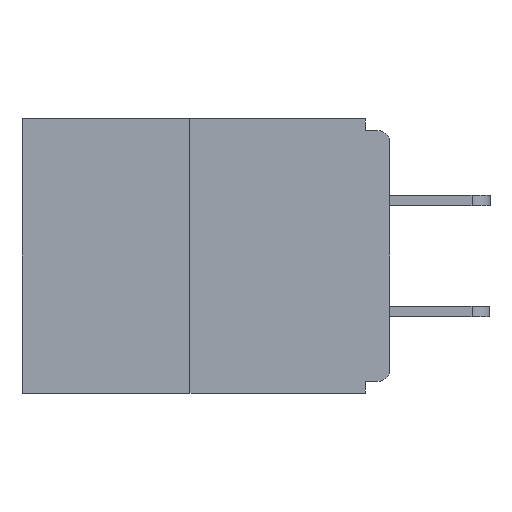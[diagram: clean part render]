
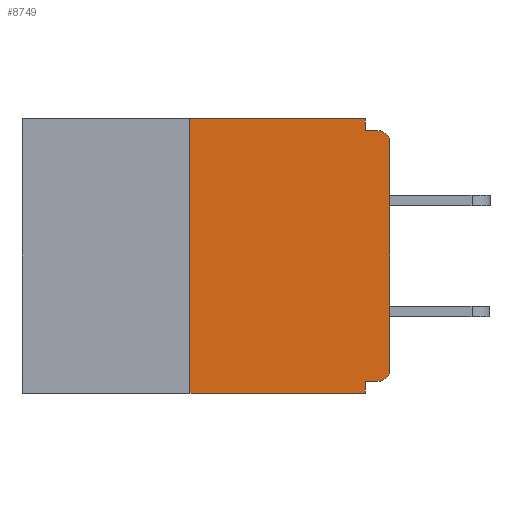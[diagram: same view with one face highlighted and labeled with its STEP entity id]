
A CAD part, left-side view. The second image highlights one B-rep face of the part: STEP entity #8749.
In plain terms, the highlighted planar face has unit normal (-1, 0, 0).
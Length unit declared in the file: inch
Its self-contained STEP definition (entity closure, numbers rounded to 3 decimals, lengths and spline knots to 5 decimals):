
#166 = DIRECTION ( 'NONE',  ( 0., -1., 0. ) ) ;
#197 = CARTESIAN_POINT ( 'NONE',  ( 0., 0.25, 0. ) ) ;
#204 = VECTOR ( 'NONE', #10966, 39.37008 ) ;
#307 = LINE ( 'NONE', #3005, #9925 ) ;
#1230 = ORIENTED_EDGE ( 'NONE', *, *, #1629, .F. ) ;
#1272 = DIRECTION ( 'NONE',  ( 0., 0., -1. ) ) ;
#1612 = ORIENTED_EDGE ( 'NONE', *, *, #14397, .F. ) ;
#1629 = EDGE_CURVE ( 'NONE', #1710, #13559, #14358, .T. ) ;
#1710 = VERTEX_POINT ( 'NONE', #3319 ) ;
#1733 = CIRCLE ( 'NONE', #5230, 0.015 ) ;
#1874 = PLANE ( 'NONE',  #7124 ) ;
#1926 = EDGE_CURVE ( 'NONE', #11104, #3265, #6083, .T. ) ;
#1977 = CARTESIAN_POINT ( 'NONE',  ( 0., 0.46, 0. ) ) ;
#2327 = CARTESIAN_POINT ( 'NONE',  ( 0., 0., -0.328 ) ) ;
#3005 = CARTESIAN_POINT ( 'NONE',  ( 0., 0., -0.015 ) ) ;
#3165 = LINE ( 'NONE', #3937, #14436 ) ;
#3265 = VERTEX_POINT ( 'NONE', #197 ) ;
#3319 = CARTESIAN_POINT ( 'NONE',  ( 0., 0.015, -0.328 ) ) ;
#3701 = DIRECTION ( 'NONE',  ( 0., 1., 0. ) ) ;
#3708 = VECTOR ( 'NONE', #14669, 39.37008 ) ;
#3818 = VECTOR ( 'NONE', #12927, 39.37008 ) ;
#3937 = CARTESIAN_POINT ( 'NONE',  ( 0., 0.46, -0.343 ) ) ;
#4058 = ORIENTED_EDGE ( 'NONE', *, *, #4877, .T. ) ;
#4300 = DIRECTION ( 'NONE',  ( 0., -1., 0. ) ) ;
#4527 = AXIS2_PLACEMENT_3D ( 'NONE', #10366, #5432, #15010 ) ;
#4700 = CARTESIAN_POINT ( 'NONE',  ( 0., 0., -0.03 ) ) ;
#4877 = EDGE_CURVE ( 'NONE', #1710, #13892, #15020, .T. ) ;
#4977 = CARTESIAN_POINT ( 'NONE',  ( 0., 0.031, 0. ) ) ;
#5230 = AXIS2_PLACEMENT_3D ( 'NONE', #10030, #14837, #7659 ) ;
#5420 = VERTEX_POINT ( 'NONE', #9673 ) ;
#5432 = DIRECTION ( 'NONE',  ( -1., 0., 0. ) ) ;
#5508 = CARTESIAN_POINT ( 'NONE',  ( 0., 0.46, 0. ) ) ;
#6083 = LINE ( 'NONE', #10564, #3818 ) ;
#6127 = CARTESIAN_POINT ( 'NONE',  ( 0., 0.031, -0.343 ) ) ;
#6521 = VERTEX_POINT ( 'NONE', #4700 ) ;
#6543 = CARTESIAN_POINT ( 'NONE',  ( 0., 0., -0.313 ) ) ;
#6548 = CARTESIAN_POINT ( 'NONE',  ( 0., 0.031, -0.328 ) ) ;
#6612 = LINE ( 'NONE', #8438, #204 ) ;
#6980 = VECTOR ( 'NONE', #1272, 39.37008 ) ;
#7124 = AXIS2_PLACEMENT_3D ( 'NONE', #5508, #13936, #10384 ) ;
#7540 = FACE_OUTER_BOUND ( 'NONE', #8474, .T. ) ;
#7659 = DIRECTION ( 'NONE',  ( 0., 0., -1. ) ) ;
#7775 = CARTESIAN_POINT ( 'NONE',  ( 0., 0.015, -0.015 ) ) ;
#8143 = EDGE_CURVE ( 'NONE', #13892, #6521, #6612, .T. ) ;
#8212 = EDGE_CURVE ( 'NONE', #13559, #14206, #12637, .T. ) ;
#8438 = CARTESIAN_POINT ( 'NONE',  ( 0., 0., 0. ) ) ;
#8474 = EDGE_LOOP ( 'NONE', ( #1612, #13403, #14239, #8706, #1230, #4058, #8990, #13829, #9928, #13115 ) ) ;
#8473 = LINE ( 'NONE', #4977, #3708 ) ;
#8488 = CARTESIAN_POINT ( 'NONE',  ( 0., 0.25, -0.343 ) ) ;
#8706 = ORIENTED_EDGE ( 'NONE', *, *, #8212, .F. ) ;
#8749 = ADVANCED_FACE ( 'NONE', ( #7540 ), #1874, .F. ) ;
#8990 = ORIENTED_EDGE ( 'NONE', *, *, #8143, .T. ) ;
#9673 = CARTESIAN_POINT ( 'NONE',  ( 0., 0.031, -0.015 ) ) ;
#9925 = VECTOR ( 'NONE', #4300, 39.37008 ) ;
#9928 = ORIENTED_EDGE ( 'NONE', *, *, #15282, .F. ) ;
#10030 = CARTESIAN_POINT ( 'NONE',  ( 0., 0.015, -0.03 ) ) ;
#10358 = EDGE_CURVE ( 'NONE', #11104, #14206, #3165, .T. ) ;
#10366 = CARTESIAN_POINT ( 'NONE',  ( 0., 0.015, -0.313 ) ) ;
#10384 = DIRECTION ( 'NONE',  ( 0., 0., -1. ) ) ;
#10564 = CARTESIAN_POINT ( 'NONE',  ( 0., 0.25, 0. ) ) ;
#10966 = DIRECTION ( 'NONE',  ( 0., 0., 1. ) ) ;
#11104 = VERTEX_POINT ( 'NONE', #8488 ) ;
#11182 = CARTESIAN_POINT ( 'NONE',  ( 0., 0.031, 0. ) ) ;
#11309 = VERTEX_POINT ( 'NONE', #7775 ) ;
#12637 = LINE ( 'NONE', #6127, #6980 ) ;
#12816 = EDGE_CURVE ( 'NONE', #6521, #11309, #1733, .T. ) ;
#12927 = DIRECTION ( 'NONE',  ( 0., 0., 1. ) ) ;
#13115 = ORIENTED_EDGE ( 'NONE', *, *, #14149, .F. ) ;
#13403 = ORIENTED_EDGE ( 'NONE', *, *, #1926, .F. ) ;
#13559 = VERTEX_POINT ( 'NONE', #6548 ) ;
#13671 = VECTOR ( 'NONE', #15181, 39.37008 ) ;
#13829 = ORIENTED_EDGE ( 'NONE', *, *, #12816, .T. ) ;
#13892 = VERTEX_POINT ( 'NONE', #6543 ) ;
#13936 = DIRECTION ( 'NONE',  ( 1., 0., 0. ) ) ;
#14149 = EDGE_CURVE ( 'NONE', #14519, #5420, #8473, .T. ) ;
#14206 = VERTEX_POINT ( 'NONE', #14914 ) ;
#14239 = ORIENTED_EDGE ( 'NONE', *, *, #10358, .T. ) ;
#14358 = LINE ( 'NONE', #2327, #14542 ) ;
#14397 = EDGE_CURVE ( 'NONE', #3265, #14519, #15543, .T. ) ;
#14436 = VECTOR ( 'NONE', #166, 39.37008 ) ;
#14519 = VERTEX_POINT ( 'NONE', #11182 ) ;
#14542 = VECTOR ( 'NONE', #3701, 39.37008 ) ;
#14669 = DIRECTION ( 'NONE',  ( 0., 0., -1. ) ) ;
#14837 = DIRECTION ( 'NONE',  ( -1., 0., 0. ) ) ;
#14914 = CARTESIAN_POINT ( 'NONE',  ( 0., 0.031, -0.343 ) ) ;
#15010 = DIRECTION ( 'NONE',  ( 0., 0., -1. ) ) ;
#15020 = CIRCLE ( 'NONE', #4527, 0.015 ) ;
#15181 = DIRECTION ( 'NONE',  ( 0., -1., 0. ) ) ;
#15282 = EDGE_CURVE ( 'NONE', #5420, #11309, #307, .T. ) ;
#15543 = LINE ( 'NONE', #1977, #13671 ) ;
